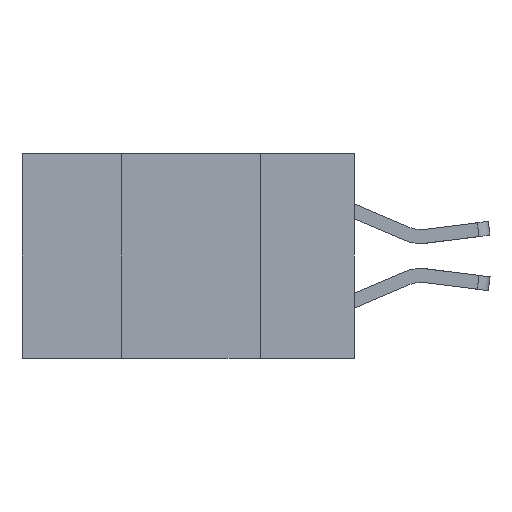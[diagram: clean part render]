
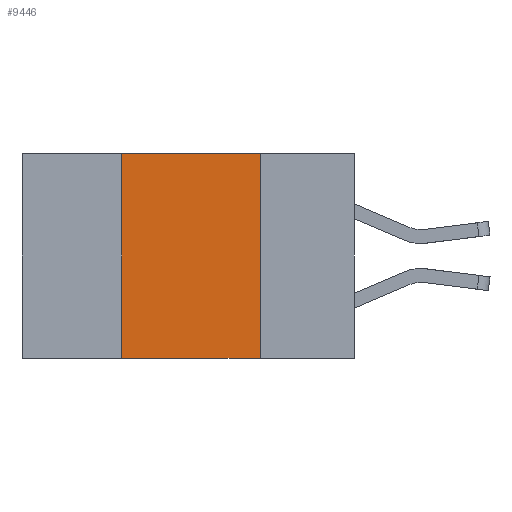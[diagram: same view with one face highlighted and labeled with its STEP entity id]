
A CAD part, left-side view. The second image highlights one B-rep face of the part: STEP entity #9446.
In plain terms, the highlighted planar face has unit normal (-1, 0, 0).
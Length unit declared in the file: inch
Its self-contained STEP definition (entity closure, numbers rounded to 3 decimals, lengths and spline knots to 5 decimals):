
#440 = DIRECTION ( 'NONE',  ( 0., 0., -1. ) ) ;
#559 = CARTESIAN_POINT ( 'NONE',  ( 0., 0.17, -0.37 ) ) ;
#693 = DIRECTION ( 'NONE',  ( 0., 0., -1. ) ) ;
#1063 = LINE ( 'NONE', #7192, #8603 ) ;
#1134 = VERTEX_POINT ( 'NONE', #2690 ) ;
#1267 = VECTOR ( 'NONE', #2826, 39.37008 ) ;
#1596 = VECTOR ( 'NONE', #2115, 39.37008 ) ;
#2115 = DIRECTION ( 'NONE',  ( 0., -1., 0. ) ) ;
#2378 = VERTEX_POINT ( 'NONE', #559 ) ;
#2669 = DIRECTION ( 'NONE',  ( 1., 0., 0. ) ) ;
#2690 = CARTESIAN_POINT ( 'NONE',  ( 0., 0.17, 0. ) ) ;
#2776 = EDGE_CURVE ( 'NONE', #5608, #8845, #1063, .T. ) ;
#2826 = DIRECTION ( 'NONE',  ( 0., -1., 0. ) ) ;
#3606 = CARTESIAN_POINT ( 'NONE',  ( 0., 0.6, 0. ) ) ;
#3607 = LINE ( 'NONE', #3606, #1596 ) ;
#3957 = LINE ( 'NONE', #6650, #5007 ) ;
#4729 = EDGE_CURVE ( 'NONE', #5608, #2378, #5527, .T. ) ;
#4730 = ORIENTED_EDGE ( 'NONE', *, *, #6168, .F. ) ;
#4999 = FACE_OUTER_BOUND ( 'NONE', #6408, .T. ) ;
#5007 = VECTOR ( 'NONE', #693, 39.37008 ) ;
#5174 = ORIENTED_EDGE ( 'NONE', *, *, #2776, .F. ) ;
#5527 = LINE ( 'NONE', #9524, #1267 ) ;
#5608 = VERTEX_POINT ( 'NONE', #5926 ) ;
#5926 = CARTESIAN_POINT ( 'NONE',  ( 0., 0.42, -0.37 ) ) ;
#6050 = AXIS2_PLACEMENT_3D ( 'NONE', #7164, #2669, #440 ) ;
#6168 = EDGE_CURVE ( 'NONE', #8845, #1134, #3607, .T. ) ;
#6386 = DIRECTION ( 'NONE',  ( 0., 0., 1. ) ) ;
#6408 = EDGE_LOOP ( 'NONE', ( #8654, #4730, #5174, #6705 ) ) ;
#6650 = CARTESIAN_POINT ( 'NONE',  ( 0., 0.17, 0. ) ) ;
#6705 = ORIENTED_EDGE ( 'NONE', *, *, #4729, .T. ) ;
#6903 = EDGE_CURVE ( 'NONE', #1134, #2378, #3957, .T. ) ;
#7164 = CARTESIAN_POINT ( 'NONE',  ( 0., 0.6, 0. ) ) ;
#7192 = CARTESIAN_POINT ( 'NONE',  ( 0., 0.42, 0. ) ) ;
#7658 = CARTESIAN_POINT ( 'NONE',  ( 0., 0.42, 0. ) ) ;
#8603 = VECTOR ( 'NONE', #6386, 39.37008 ) ;
#8654 = ORIENTED_EDGE ( 'NONE', *, *, #6903, .F. ) ;
#8845 = VERTEX_POINT ( 'NONE', #7658 ) ;
#9438 = PLANE ( 'NONE',  #6050 ) ;
#9446 = ADVANCED_FACE ( 'NONE', ( #4999 ), #9438, .F. ) ;
#9524 = CARTESIAN_POINT ( 'NONE',  ( 0., 0.6, -0.37 ) ) ;
